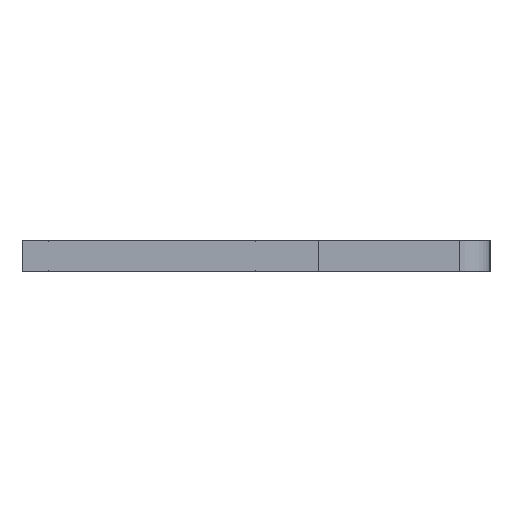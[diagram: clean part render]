
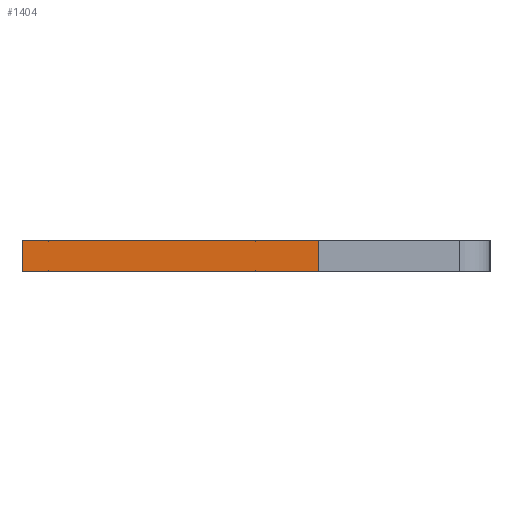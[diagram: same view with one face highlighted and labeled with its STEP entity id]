
A CAD part, left-side view. The second image highlights one B-rep face of the part: STEP entity #1404.
In plain terms, the highlighted face is planar.
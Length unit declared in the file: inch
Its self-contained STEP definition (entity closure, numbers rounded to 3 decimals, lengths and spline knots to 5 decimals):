
#30 = CARTESIAN_POINT ( 'NONE',  ( -0.01, 0.15, -0.04 ) ) ;
#182 = CARTESIAN_POINT ( 'NONE',  ( 0.01, 0.15, -0.04 ) ) ;
#221 = VECTOR ( 'NONE', #444, 39.37008 ) ;
#354 = FACE_OUTER_BOUND ( 'NONE', #1599, .T. ) ;
#444 = DIRECTION ( 'NONE',  ( 0., 1., 0. ) ) ;
#450 = ORIENTED_EDGE ( 'NONE', *, *, #2795, .F. ) ;
#526 = CARTESIAN_POINT ( 'NONE',  ( 0.01, 0.15, -0.04 ) ) ;
#563 = LINE ( 'NONE', #182, #1037 ) ;
#632 = VERTEX_POINT ( 'NONE', #1174 ) ;
#770 = DIRECTION ( 'NONE',  ( 0., 0., 1. ) ) ;
#994 = CARTESIAN_POINT ( 'NONE',  ( 0.01, 0.15, -0.04 ) ) ;
#1037 = VECTOR ( 'NONE', #1517, 39.37008 ) ;
#1057 = ORIENTED_EDGE ( 'NONE', *, *, #1167, .F. ) ;
#1167 = EDGE_CURVE ( 'NONE', #1638, #1579, #563, .T. ) ;
#1174 = CARTESIAN_POINT ( 'NONE',  ( -0.01, -0.04, -0.04 ) ) ;
#1290 = DIRECTION ( 'NONE',  ( 1., 0., 0. ) ) ;
#1404 = ADVANCED_FACE ( 'NONE', ( #354 ), #2586, .F. ) ;
#1517 = DIRECTION ( 'NONE',  ( -1., 0., 0. ) ) ;
#1523 = DIRECTION ( 'NONE',  ( -1., 0., 0. ) ) ;
#1579 = VERTEX_POINT ( 'NONE', #3094 ) ;
#1599 = EDGE_LOOP ( 'NONE', ( #1675, #1057, #450, #2009 ) ) ;
#1637 = CARTESIAN_POINT ( 'NONE',  ( 0.01, -0.04, -0.04 ) ) ;
#1638 = VERTEX_POINT ( 'NONE', #526 ) ;
#1670 = VERTEX_POINT ( 'NONE', #1637 ) ;
#1675 = ORIENTED_EDGE ( 'NONE', *, *, #1910, .T. ) ;
#1685 = LINE ( 'NONE', #994, #221 ) ;
#1910 = EDGE_CURVE ( 'NONE', #632, #1579, #2246, .T. ) ;
#2009 = ORIENTED_EDGE ( 'NONE', *, *, #2188, .T. ) ;
#2142 = LINE ( 'NONE', #3040, #2416 ) ;
#2188 = EDGE_CURVE ( 'NONE', #1670, #632, #2142, .T. ) ;
#2246 = LINE ( 'NONE', #30, #3068 ) ;
#2416 = VECTOR ( 'NONE', #1523, 39.37008 ) ;
#2451 = AXIS2_PLACEMENT_3D ( 'NONE', #2614, #770, #1290 ) ;
#2586 = PLANE ( 'NONE',  #2451 ) ;
#2614 = CARTESIAN_POINT ( 'NONE',  ( 0.01, 0.15, -0.04 ) ) ;
#2795 = EDGE_CURVE ( 'NONE', #1670, #1638, #1685, .T. ) ;
#2948 = DIRECTION ( 'NONE',  ( 0., 1., 0. ) ) ;
#3040 = CARTESIAN_POINT ( 'NONE',  ( 0.01, -0.04, -0.04 ) ) ;
#3068 = VECTOR ( 'NONE', #2948, 39.37008 ) ;
#3094 = CARTESIAN_POINT ( 'NONE',  ( -0.01, 0.15, -0.04 ) ) ;
